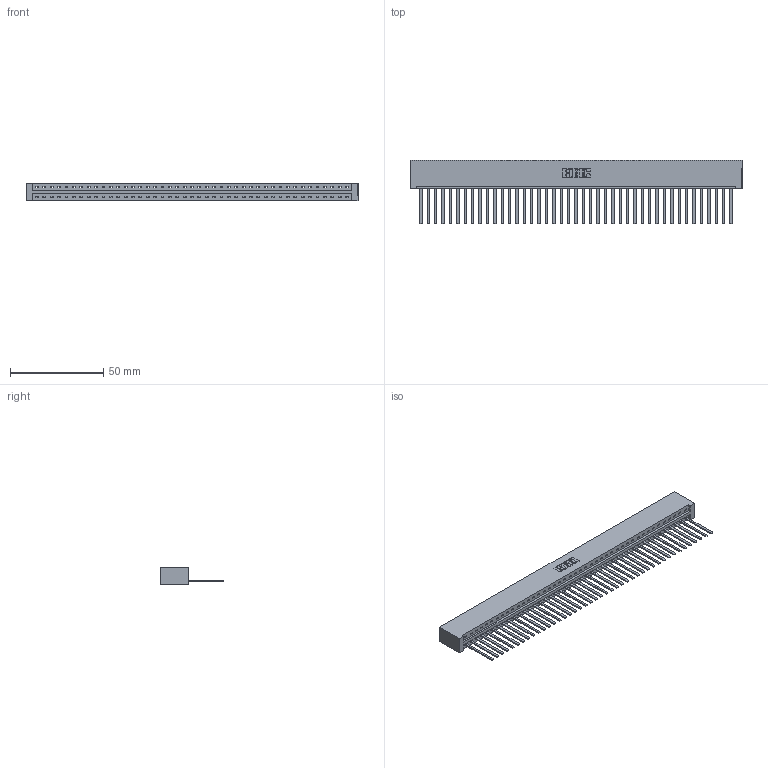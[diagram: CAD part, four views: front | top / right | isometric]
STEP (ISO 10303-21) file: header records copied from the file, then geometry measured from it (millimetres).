
FILE_DESCRIPTION (( 'STEP AP203' ), '1' );
FILE_NAME ('337-043-544-101.STEP', '2019-10-01T23:58:43', ( '' ), ( '' ), 'SwSTEP 2.0', 'SolidWorks 2016', '' );
FILE_SCHEMA (( 'CONFIG_CONTROL_DESIGN' ));
Length unit declared in the file: inch
Products named in the file (3): 337 Part_No Mounting Lugs; 345-292-001_345-293-144; 337-043-544-101
Assembly tree (44 placements, depth 2):
  337-043-544-101
    337 Part_No Mounting Lugs
    345-292-001_345-293-144  x43
Bounding box: 178.26 x 34.3 x 9.4 mm (x, y, z)
Volume: 19776.1 mm3; surface area: 22060.8 mm2
Topology: 44 solids, 44 shells, 2514 faces, 7597 edges, 5006 vertices
Faces by surface type: plane 1872, cylinder 642
Entity records: 31373 total; most frequent: CARTESIAN_POINT 5471, ORIENTED_EDGE 5450, DIRECTION 4591, EDGE_CURVE 2725, LINE 2609, VECTOR 2609, VERTEX_POINT 1814, AXIS2_PLACEMENT_3D 991
